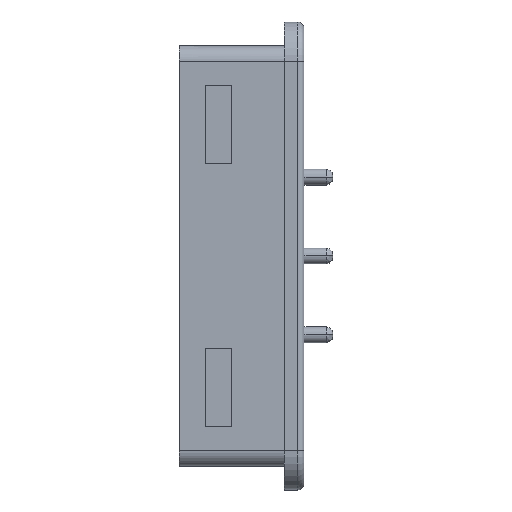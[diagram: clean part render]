
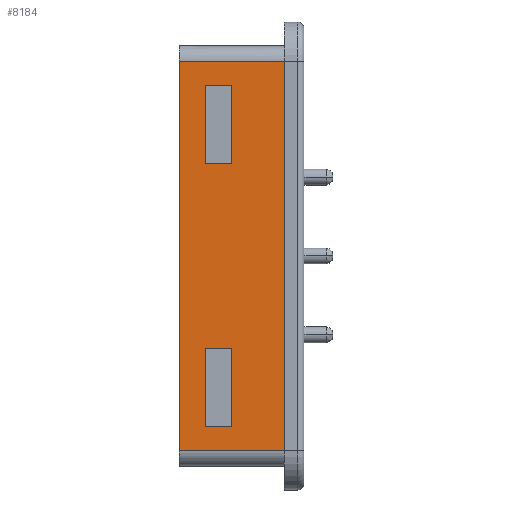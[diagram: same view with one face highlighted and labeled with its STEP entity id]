
A CAD part, left-side view. The second image highlights one B-rep face of the part: STEP entity #8184.
In plain terms, the highlighted planar face has unit normal (-1, 0, 0).
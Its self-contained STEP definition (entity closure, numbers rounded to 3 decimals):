
#203 = VERTEX_POINT ( 'NONE', #10158 ) ;
#341 = FACE_BOUND ( 'NONE', #8533, .T. ) ;
#689 = CARTESIAN_POINT ( 'NONE',  ( -8.5, 5.5, -13. ) ) ;
#724 = LINE ( 'NONE', #4026, #1012 ) ;
#912 = CARTESIAN_POINT ( 'NONE',  ( -8.5, 7.5, 13. ) ) ;
#1012 = VECTOR ( 'NONE', #7318, 1000. ) ;
#1196 = VERTEX_POINT ( 'NONE', #7715 ) ;
#1296 = DIRECTION ( 'NONE',  ( 0., -1., 0. ) ) ;
#1670 = EDGE_CURVE ( 'NONE', #3598, #9940, #6986, .T. ) ;
#1673 = LINE ( 'NONE', #4951, #5198 ) ;
#1880 = ORIENTED_EDGE ( 'NONE', *, *, #4153, .F. ) ;
#1930 = CARTESIAN_POINT ( 'NONE',  ( -8.5, 9.5, -14.8 ) ) ;
#2012 = ORIENTED_EDGE ( 'NONE', *, *, #6773, .T. ) ;
#2017 = CARTESIAN_POINT ( 'NONE',  ( -8.5, 9.5, -14.8 ) ) ;
#2059 = ORIENTED_EDGE ( 'NONE', *, *, #4283, .T. ) ;
#2120 = CARTESIAN_POINT ( 'NONE',  ( -8.5, 7.5, 7. ) ) ;
#2179 = VERTEX_POINT ( 'NONE', #3904 ) ;
#2191 = EDGE_CURVE ( 'NONE', #203, #7955, #7191, .T. ) ;
#2220 = CARTESIAN_POINT ( 'NONE',  ( -8.5, 5.5, 13. ) ) ;
#2245 = CARTESIAN_POINT ( 'NONE',  ( -8.5, 9.5, 14.8 ) ) ;
#2267 = EDGE_LOOP ( 'NONE', ( #2775, #1880, #10095, #6207 ) ) ;
#2742 = DIRECTION ( 'NONE',  ( 0., -1., 0. ) ) ;
#2775 = ORIENTED_EDGE ( 'NONE', *, *, #1670, .T. ) ;
#2833 = DIRECTION ( 'NONE',  ( 1., 0., 0. ) ) ;
#2890 = DIRECTION ( 'NONE',  ( 0., 1., 0. ) ) ;
#3051 = VECTOR ( 'NONE', #1296, 1000. ) ;
#3093 = DIRECTION ( 'NONE',  ( 0., 0., -1. ) ) ;
#3163 = LINE ( 'NONE', #6461, #4436 ) ;
#3193 = CARTESIAN_POINT ( 'NONE',  ( -8.5, 1.5, -14.8 ) ) ;
#3404 = AXIS2_PLACEMENT_3D ( 'NONE', #10239, #2833, #6115 ) ;
#3537 = EDGE_CURVE ( 'NONE', #9638, #9258, #9523, .T. ) ;
#3598 = VERTEX_POINT ( 'NONE', #3838 ) ;
#3644 = FACE_BOUND ( 'NONE', #5939, .T. ) ;
#3838 = CARTESIAN_POINT ( 'NONE',  ( -8.5, 1.5, 14.8 ) ) ;
#3904 = CARTESIAN_POINT ( 'NONE',  ( -8.5, 1.5, -14.8 ) ) ;
#3996 = DIRECTION ( 'NONE',  ( 0., 1., 0. ) ) ;
#4017 = EDGE_CURVE ( 'NONE', #9481, #1196, #9616, .T. ) ;
#4026 = CARTESIAN_POINT ( 'NONE',  ( -8.5, 7.5, -13. ) ) ;
#4153 = EDGE_CURVE ( 'NONE', #9813, #9940, #1673, .T. ) ;
#4241 = CARTESIAN_POINT ( 'NONE',  ( -8.5, 7.5, 7. ) ) ;
#4283 = EDGE_CURVE ( 'NONE', #9258, #9481, #6835, .T. ) ;
#4436 = VECTOR ( 'NONE', #9769, 1000. ) ;
#4951 = CARTESIAN_POINT ( 'NONE',  ( -8.5, 9.5, -14.8 ) ) ;
#5170 = VERTEX_POINT ( 'NONE', #10369 ) ;
#5198 = VECTOR ( 'NONE', #8271, 1000. ) ;
#5211 = DIRECTION ( 'NONE',  ( 0., -1., 0. ) ) ;
#5368 = VECTOR ( 'NONE', #2890, 1000. ) ;
#5391 = LINE ( 'NONE', #8702, #3051 ) ;
#5400 = DIRECTION ( 'NONE',  ( 0., 0., 1. ) ) ;
#5493 = DIRECTION ( 'NONE',  ( 0., 0., -1. ) ) ;
#5928 = VECTOR ( 'NONE', #3093, 1000. ) ;
#5939 = EDGE_LOOP ( 'NONE', ( #7090, #2059, #8880, #2012 ) ) ;
#6115 = DIRECTION ( 'NONE',  ( 0., 1., 0. ) ) ;
#6207 = ORIENTED_EDGE ( 'NONE', *, *, #8779, .T. ) ;
#6283 = EDGE_CURVE ( 'NONE', #5170, #203, #5391, .T. ) ;
#6343 = CARTESIAN_POINT ( 'NONE',  ( -8.5, 5.5, 13. ) ) ;
#6410 = EDGE_CURVE ( 'NONE', #7955, #9529, #8118, .T. ) ;
#6461 = CARTESIAN_POINT ( 'NONE',  ( -8.5, 5.5, 7. ) ) ;
#6488 = DIRECTION ( 'NONE',  ( 0., 0., 1. ) ) ;
#6747 = VECTOR ( 'NONE', #5493, 1000. ) ;
#6773 = EDGE_CURVE ( 'NONE', #1196, #9638, #3163, .T. ) ;
#6835 = LINE ( 'NONE', #10146, #6921 ) ;
#6852 = VECTOR ( 'NONE', #5211, 1000. ) ;
#6921 = VECTOR ( 'NONE', #2742, 1000. ) ;
#6933 = PLANE ( 'NONE',  #3404 ) ;
#6986 = LINE ( 'NONE', #10296, #5368 ) ;
#7045 = EDGE_CURVE ( 'NONE', #9813, #2179, #9332, .T. ) ;
#7090 = ORIENTED_EDGE ( 'NONE', *, *, #3537, .T. ) ;
#7191 = LINE ( 'NONE', #10504, #5928 ) ;
#7255 = EDGE_CURVE ( 'NONE', #9529, #5170, #724, .T. ) ;
#7318 = DIRECTION ( 'NONE',  ( 0., 0., 1. ) ) ;
#7715 = CARTESIAN_POINT ( 'NONE',  ( -8.5, 5.5, 7. ) ) ;
#7747 = FACE_OUTER_BOUND ( 'NONE', #2267, .T. ) ;
#7955 = VERTEX_POINT ( 'NONE', #8209 ) ;
#8074 = VECTOR ( 'NONE', #3996, 1000. ) ;
#8118 = LINE ( 'NONE', #689, #8074 ) ;
#8184 = ADVANCED_FACE ( 'NONE', ( #7747, #341, #3644 ), #6933, .F. ) ;
#8209 = CARTESIAN_POINT ( 'NONE',  ( -8.5, 5.5, -13. ) ) ;
#8271 = DIRECTION ( 'NONE',  ( 0., 0., 1. ) ) ;
#8533 = EDGE_LOOP ( 'NONE', ( #8648, #10177, #9409, #9220 ) ) ;
#8648 = ORIENTED_EDGE ( 'NONE', *, *, #6283, .T. ) ;
#8702 = CARTESIAN_POINT ( 'NONE',  ( -8.5, 7.5, -7. ) ) ;
#8779 = EDGE_CURVE ( 'NONE', #2179, #3598, #10609, .T. ) ;
#8880 = ORIENTED_EDGE ( 'NONE', *, *, #4017, .T. ) ;
#9220 = ORIENTED_EDGE ( 'NONE', *, *, #7255, .T. ) ;
#9258 = VERTEX_POINT ( 'NONE', #912 ) ;
#9332 = LINE ( 'NONE', #1930, #6852 ) ;
#9393 = VECTOR ( 'NONE', #6488, 1000. ) ;
#9409 = ORIENTED_EDGE ( 'NONE', *, *, #6410, .T. ) ;
#9481 = VERTEX_POINT ( 'NONE', #6343 ) ;
#9523 = LINE ( 'NONE', #2120, #10549 ) ;
#9529 = VERTEX_POINT ( 'NONE', #9762 ) ;
#9616 = LINE ( 'NONE', #2220, #6747 ) ;
#9638 = VERTEX_POINT ( 'NONE', #4241 ) ;
#9762 = CARTESIAN_POINT ( 'NONE',  ( -8.5, 7.5, -13. ) ) ;
#9769 = DIRECTION ( 'NONE',  ( 0., 1., 0. ) ) ;
#9813 = VERTEX_POINT ( 'NONE', #2017 ) ;
#9940 = VERTEX_POINT ( 'NONE', #2245 ) ;
#10095 = ORIENTED_EDGE ( 'NONE', *, *, #7045, .T. ) ;
#10146 = CARTESIAN_POINT ( 'NONE',  ( -8.5, 7.5, 13. ) ) ;
#10158 = CARTESIAN_POINT ( 'NONE',  ( -8.5, 5.5, -7. ) ) ;
#10177 = ORIENTED_EDGE ( 'NONE', *, *, #2191, .T. ) ;
#10239 = CARTESIAN_POINT ( 'NONE',  ( -8.5, 5.5, 0. ) ) ;
#10296 = CARTESIAN_POINT ( 'NONE',  ( -8.5, 1.5, 14.8 ) ) ;
#10369 = CARTESIAN_POINT ( 'NONE',  ( -8.5, 7.5, -7. ) ) ;
#10504 = CARTESIAN_POINT ( 'NONE',  ( -8.5, 5.5, -7. ) ) ;
#10549 = VECTOR ( 'NONE', #5400, 1000. ) ;
#10609 = LINE ( 'NONE', #3193, #9393 ) ;
